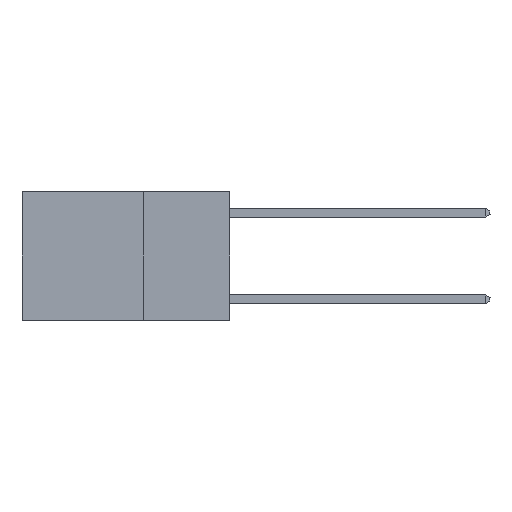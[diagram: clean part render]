
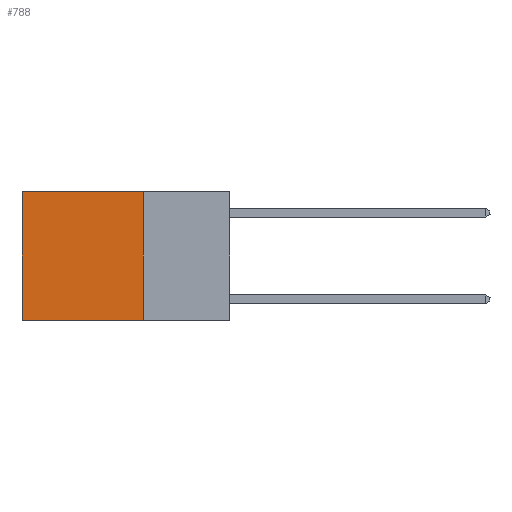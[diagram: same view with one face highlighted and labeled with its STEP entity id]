
A CAD part, left-side view. The second image highlights one B-rep face of the part: STEP entity #788.
In plain terms, the highlighted planar face has unit normal (-1, 0, 0).
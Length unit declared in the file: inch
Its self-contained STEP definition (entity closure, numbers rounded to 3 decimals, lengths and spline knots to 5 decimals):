
#591 = ORIENTED_EDGE ( 'NONE', *, *, #11470, .F. ) ;
#788 = ADVANCED_FACE ( 'NONE', ( #6021 ), #4497, .F. ) ;
#1225 = LINE ( 'NONE', #13318, #8384 ) ;
#1953 = LINE ( 'NONE', #15542, #12943 ) ;
#3029 = DIRECTION ( 'NONE',  ( 1., 0., 0. ) ) ;
#3155 = ORIENTED_EDGE ( 'NONE', *, *, #18121, .T. ) ;
#3689 = LINE ( 'NONE', #5485, #13882 ) ;
#3850 = CARTESIAN_POINT ( 'NONE',  ( 0.2625, 0.25, -0.37 ) ) ;
#3885 = VECTOR ( 'NONE', #9881, 39.37008 ) ;
#4497 = PLANE ( 'NONE',  #7153 ) ;
#5485 = CARTESIAN_POINT ( 'NONE',  ( 0.2625, 0.25, 0. ) ) ;
#5703 = EDGE_CURVE ( 'NONE', #15732, #12801, #1953, .T. ) ;
#6021 = FACE_OUTER_BOUND ( 'NONE', #6392, .T. ) ;
#6253 = ORIENTED_EDGE ( 'NONE', *, *, #6614, .T. ) ;
#6392 = EDGE_LOOP ( 'NONE', ( #3155, #7336, #591, #6253 ) ) ;
#6614 = EDGE_CURVE ( 'NONE', #16616, #15883, #3689, .T. ) ;
#7078 = DIRECTION ( 'NONE',  ( 0., 1., 0. ) ) ;
#7153 = AXIS2_PLACEMENT_3D ( 'NONE', #16609, #3029, #9074 ) ;
#7336 = ORIENTED_EDGE ( 'NONE', *, *, #5703, .F. ) ;
#8027 = DIRECTION ( 'NONE',  ( 0., 1., 0. ) ) ;
#8384 = VECTOR ( 'NONE', #17873, 39.37008 ) ;
#9074 = DIRECTION ( 'NONE',  ( 0., 0., -1. ) ) ;
#9881 = DIRECTION ( 'NONE',  ( 0., 0., -1. ) ) ;
#10179 = CARTESIAN_POINT ( 'NONE',  ( 0.2625, 0.6, -0.37 ) ) ;
#11470 = EDGE_CURVE ( 'NONE', #16616, #15732, #13053, .T. ) ;
#12801 = VERTEX_POINT ( 'NONE', #10179 ) ;
#12943 = VECTOR ( 'NONE', #8027, 39.37008 ) ;
#13053 = LINE ( 'NONE', #19196, #3885 ) ;
#13318 = CARTESIAN_POINT ( 'NONE',  ( 0.2625, 0.6, 0. ) ) ;
#13882 = VECTOR ( 'NONE', #7078, 39.37008 ) ;
#14653 = CARTESIAN_POINT ( 'NONE',  ( 0.2625, 0.6, 0. ) ) ;
#15542 = CARTESIAN_POINT ( 'NONE',  ( 0.2625, 0.25, -0.37 ) ) ;
#15732 = VERTEX_POINT ( 'NONE', #3850 ) ;
#15883 = VERTEX_POINT ( 'NONE', #14653 ) ;
#16609 = CARTESIAN_POINT ( 'NONE',  ( 0.2625, 0.25, 0. ) ) ;
#16616 = VERTEX_POINT ( 'NONE', #18874 ) ;
#17873 = DIRECTION ( 'NONE',  ( 0., 0., -1. ) ) ;
#18121 = EDGE_CURVE ( 'NONE', #15883, #12801, #1225, .T. ) ;
#18874 = CARTESIAN_POINT ( 'NONE',  ( 0.2625, 0.25, 0. ) ) ;
#19196 = CARTESIAN_POINT ( 'NONE',  ( 0.2625, 0.25, 0. ) ) ;
